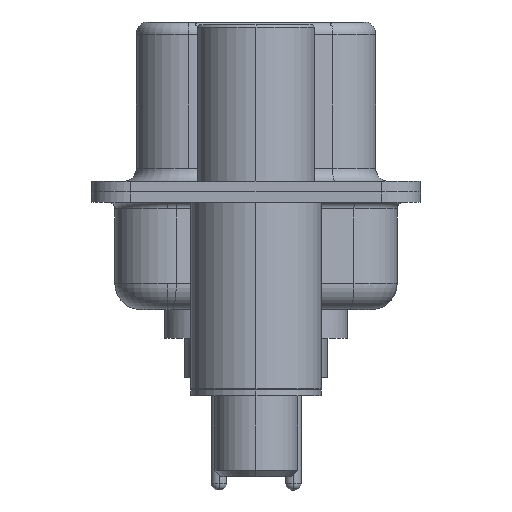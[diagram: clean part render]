
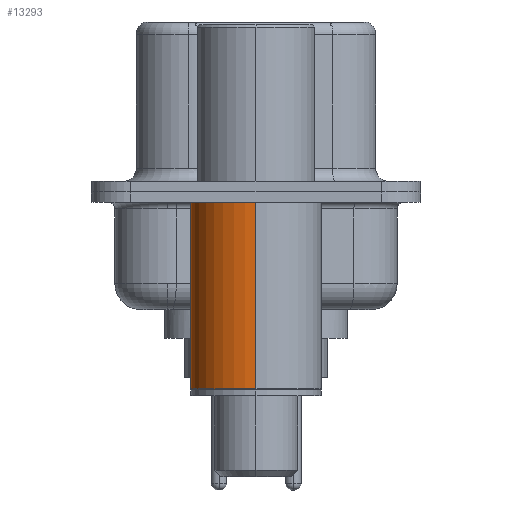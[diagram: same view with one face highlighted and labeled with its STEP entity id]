
A CAD part, left-side view. The second image highlights one B-rep face of the part: STEP entity #13293.
In plain terms, the highlighted cylindrical face has radius 2.5 mm (diameter 5 mm), a partial arc.
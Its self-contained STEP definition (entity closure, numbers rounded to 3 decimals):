
#1362 = EDGE_CURVE ( 'NONE', #21987, #13460, #14557, .T. ) ;
#1407 = DIRECTION ( 'NONE',  ( 0., 0., 1. ) ) ;
#1934 = CIRCLE ( 'NONE', #4465, 2.5 ) ;
#2018 = CIRCLE ( 'NONE', #8015, 2.5 ) ;
#2894 = AXIS2_PLACEMENT_3D ( 'NONE', #5661, #25034, #11507 ) ;
#3351 = ORIENTED_EDGE ( 'NONE', *, *, #1362, .F. ) ;
#4230 = VECTOR ( 'NONE', #11651, 1000. ) ;
#4465 = AXIS2_PLACEMENT_3D ( 'NONE', #15437, #12232, #12320 ) ;
#5661 = CARTESIAN_POINT ( 'NONE',  ( 0., 0., 0.581 ) ) ;
#5775 = EDGE_CURVE ( 'NONE', #13460, #8303, #1934, .T. ) ;
#7205 = VECTOR ( 'NONE', #24076, 1000. ) ;
#8015 = AXIS2_PLACEMENT_3D ( 'NONE', #13096, #1407, #15029 ) ;
#8303 = VERTEX_POINT ( 'NONE', #16999 ) ;
#10281 = CARTESIAN_POINT ( 'NONE',  ( 2.5, 0., -7.525 ) ) ;
#11507 = DIRECTION ( 'NONE',  ( 1., 0., 0. ) ) ;
#11651 = DIRECTION ( 'NONE',  ( 0., 0., 1. ) ) ;
#12232 = DIRECTION ( 'NONE',  ( 0., 0., 1. ) ) ;
#12320 = DIRECTION ( 'NONE',  ( 1., 0., 0. ) ) ;
#12354 = VERTEX_POINT ( 'NONE', #19856 ) ;
#13096 = CARTESIAN_POINT ( 'NONE',  ( 0., 0., -7.525 ) ) ;
#13293 = ADVANCED_FACE ( 'NONE', ( #25057 ), #14767, .T. ) ;
#13460 = VERTEX_POINT ( 'NONE', #23633 ) ;
#13467 = ORIENTED_EDGE ( 'NONE', *, *, #5775, .F. ) ;
#13536 = ORIENTED_EDGE ( 'NONE', *, *, #17956, .T. ) ;
#13579 = LINE ( 'NONE', #20180, #7205 ) ;
#13877 = ORIENTED_EDGE ( 'NONE', *, *, #18433, .T. ) ;
#14557 = LINE ( 'NONE', #15870, #4230 ) ;
#14767 = CYLINDRICAL_SURFACE ( 'NONE', #2894, 2.5 ) ;
#15029 = DIRECTION ( 'NONE',  ( 1., 0., 0. ) ) ;
#15437 = CARTESIAN_POINT ( 'NONE',  ( 0., 0., -0.4 ) ) ;
#15870 = CARTESIAN_POINT ( 'NONE',  ( 2.5, 0., 0.581 ) ) ;
#16999 = CARTESIAN_POINT ( 'NONE',  ( -2.5, 0., -0.4 ) ) ;
#17956 = EDGE_CURVE ( 'NONE', #21987, #12354, #2018, .T. ) ;
#18433 = EDGE_CURVE ( 'NONE', #12354, #8303, #13579, .T. ) ;
#19856 = CARTESIAN_POINT ( 'NONE',  ( -2.5, 0., -7.525 ) ) ;
#20091 = EDGE_LOOP ( 'NONE', ( #13536, #13877, #13467, #3351 ) ) ;
#20180 = CARTESIAN_POINT ( 'NONE',  ( -2.5, 0., 0.581 ) ) ;
#21987 = VERTEX_POINT ( 'NONE', #10281 ) ;
#23633 = CARTESIAN_POINT ( 'NONE',  ( 2.5, 0., -0.4 ) ) ;
#24076 = DIRECTION ( 'NONE',  ( 0., 0., 1. ) ) ;
#25034 = DIRECTION ( 'NONE',  ( 0., 0., 1. ) ) ;
#25057 = FACE_OUTER_BOUND ( 'NONE', #20091, .T. ) ;
